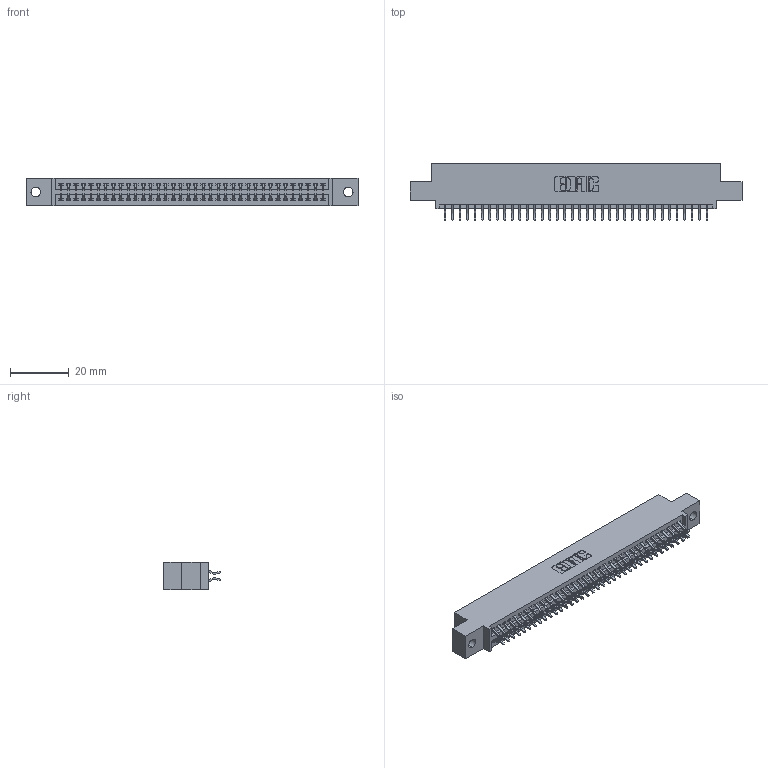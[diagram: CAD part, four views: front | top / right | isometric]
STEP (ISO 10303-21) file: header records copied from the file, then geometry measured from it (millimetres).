
FILE_DESCRIPTION (( 'STEP AP203' ), '1' );
FILE_NAME ('345-072-556-502.STEP', '2019-10-31T04:29:46', ( '' ), ( '' ), 'SwSTEP 2.0', 'SolidWorks 2016', '' );
FILE_SCHEMA (( 'CONFIG_CONTROL_DESIGN' ));
Length unit declared in the file: inch
Products named in the file (3): 345-292-001_556 Tail; 345-072-556-502; 345 Part_0.110 Offset - 0.128 Dia
Assembly tree (73 placements, depth 2):
  345-072-556-502
    345 Part_0.110 Offset - 0.128 Dia
    345-292-001_556 Tail  x72
Bounding box: 112.65 x 19.24 x 9.4 mm (x, y, z)
Volume: 10774.2 mm3; surface area: 15567 mm2
Topology: 73 solids, 73 shells, 4162 faces, 12377 edges, 8154 vertices
Faces by surface type: plane 2748, cylinder 1414
Entity records: 29409 total; most frequent: CARTESIAN_POINT 4952, ORIENTED_EDGE 4874, DIRECTION 4361, EDGE_CURVE 2437, VECTOR 2153, LINE 2153, VERTEX_POINT 1622, AXIS2_PLACEMENT_3D 1104
